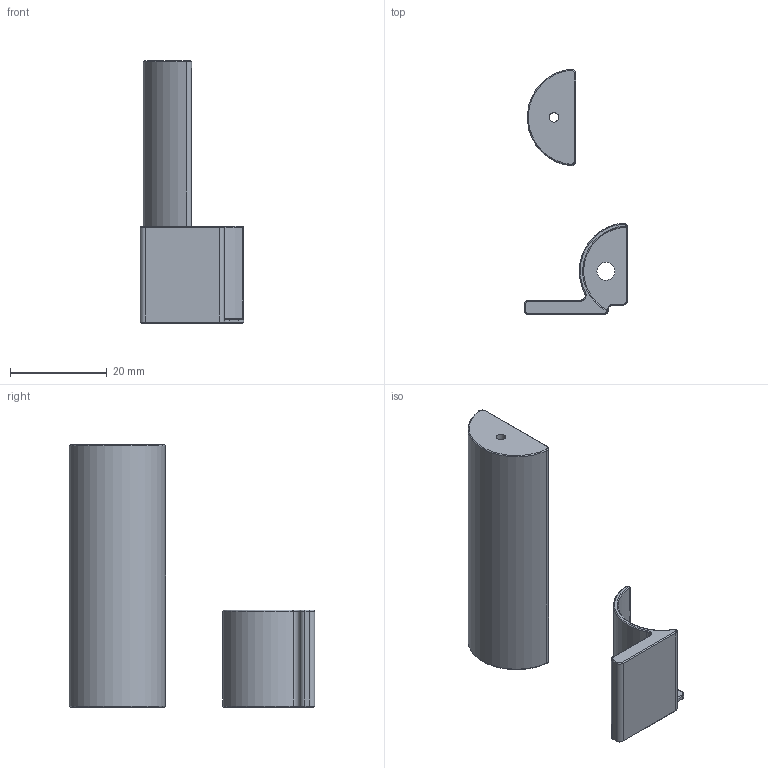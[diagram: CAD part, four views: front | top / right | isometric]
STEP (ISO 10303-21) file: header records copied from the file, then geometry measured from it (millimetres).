
FILE_DESCRIPTION(/* description */ (''),/* implementation_level */ '2;1');
FILE_NAME(/* name */ 'FGC-9_Bolt_Jigs.step',/* time_stamp */ '2020-03-26T20:08:58+01:00',/* author */ (''),/* organization */ (''),/* preprocessor_version */ 'ST-DEVELOPER v18',/* originating_system */ 'Autodesk Translation Framework v8.12.0.6',/* authorisation */ '');
FILE_SCHEMA (('AUTOMOTIVE_DESIGN { 1 0 10303 214 3 1 1 }'));
Length unit declared in the file: millimetre
Products named in the file (3): FGC-9 Bolt Jigs; Drilling Jig; Welding Jig
Assembly tree (2 placements, depth 2):
  FGC-9 Bolt Jigs
    Drilling Jig
    Welding Jig
Bounding box: 21.37 x 50.69 x 54.15 mm (x, y, z)
Volume: 3372.5 mm3; surface area: 5733.7 mm2
Topology: 2 solids, 2 shells, 79 faces, 182 edges, 106 vertices
Faces by surface type: cylinder 34, torus 29, plane 14, sphere 2
Full cylindrical faces by diameter (mm): 2 x2, 3.7 x1
Entity records: 2413 total; most frequent: CARTESIAN_POINT 462, DIRECTION 458, ORIENTED_EDGE 362, AXIS2_PLACEMENT_3D 200, EDGE_CURVE 181, CIRCLE 116, VERTEX_POINT 106, EDGE_LOOP 85
